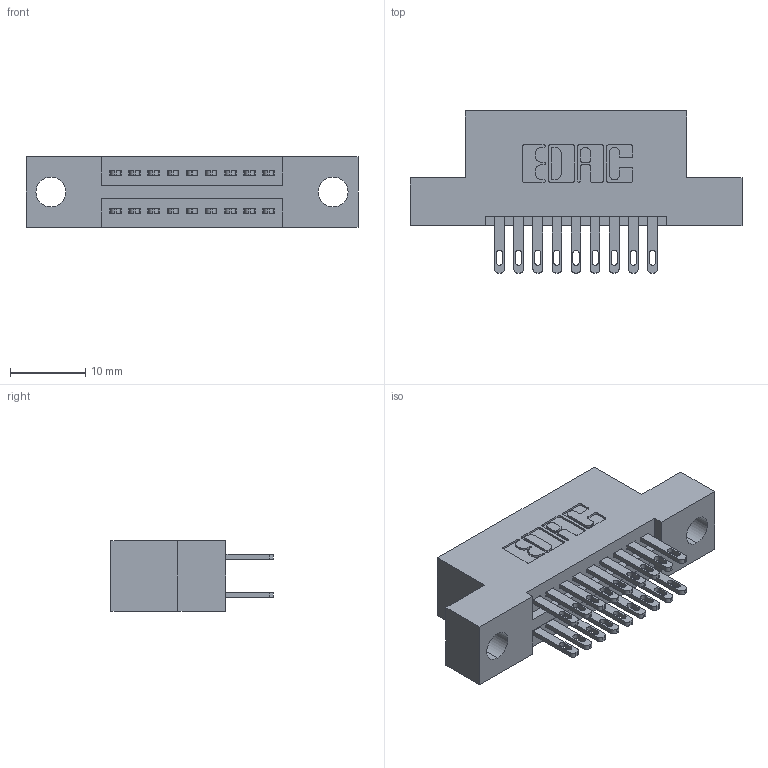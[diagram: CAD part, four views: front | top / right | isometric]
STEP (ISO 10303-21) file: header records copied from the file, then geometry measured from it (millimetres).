
FILE_DESCRIPTION (( 'STEP AP203' ), '1' );
FILE_NAME ('895-018-500-204.STEP', '2020-09-25T06:00:09', ( '' ), ( '' ), 'SwSTEP 2.0', 'SolidWorks 2020', '' );
FILE_SCHEMA (( 'CONFIG_CONTROL_DESIGN' ));
Length unit declared in the file: inch
Products named in the file (3): 845 Part_Flush Mounting Lugs - 0.156 Dia-TH; 345-292-001_345-293-100; 895-018-500-204
Assembly tree (19 placements, depth 2):
  895-018-500-204
    845 Part_Flush Mounting Lugs - 0.156 Dia-TH
    345-292-001_345-293-100  x18
Bounding box: 44.07 x 21.51 x 9.4 mm (x, y, z)
Volume: 3941.7 mm3; surface area: 5186.2 mm2
Topology: 19 solids, 19 shells, 954 faces, 2879 edges, 1918 vertices
Faces by surface type: plane 566, cylinder 388
Entity records: 11437 total; most frequent: CARTESIAN_POINT 1948, ORIENTED_EDGE 1882, DIRECTION 1761, EDGE_CURVE 941, VECTOR 769, LINE 769, VERTEX_POINT 626, AXIS2_PLACEMENT_3D 496
